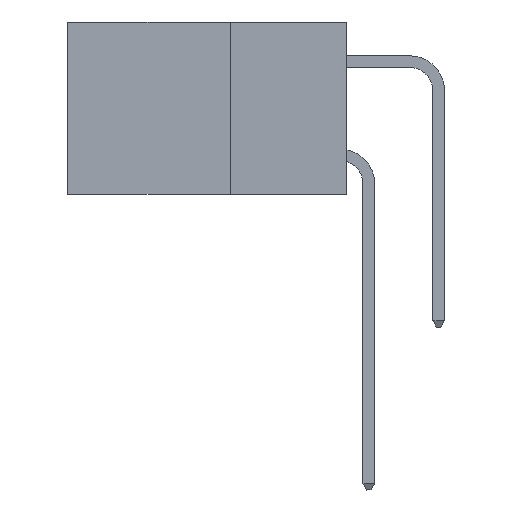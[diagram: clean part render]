
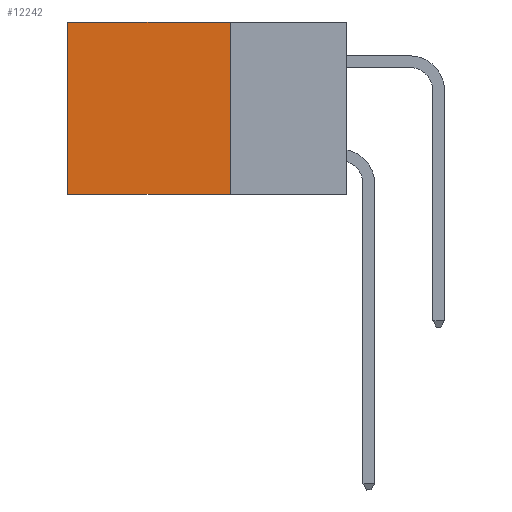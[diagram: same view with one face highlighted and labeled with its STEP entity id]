
A CAD part, left-side view. The second image highlights one B-rep face of the part: STEP entity #12242.
In plain terms, the highlighted planar face has unit normal (-1, 0, 0).
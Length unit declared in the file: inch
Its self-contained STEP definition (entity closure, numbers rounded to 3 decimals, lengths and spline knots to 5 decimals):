
#131 = VERTEX_POINT ( 'NONE', #12599 ) ;
#563 = CARTESIAN_POINT ( 'NONE',  ( 0.2875, 0.25, 0. ) ) ;
#2231 = EDGE_CURVE ( 'NONE', #131, #17688, #21309, .T. ) ;
#2448 = CARTESIAN_POINT ( 'NONE',  ( 0.2875, 0.6, 0. ) ) ;
#2925 = DIRECTION ( 'NONE',  ( 1., 0., 0. ) ) ;
#4211 = CARTESIAN_POINT ( 'NONE',  ( 0.2875, 0.25, -0.37 ) ) ;
#4429 = DIRECTION ( 'NONE',  ( 0., 1., 0. ) ) ;
#4954 = CARTESIAN_POINT ( 'NONE',  ( 0.2875, 0.6, 0. ) ) ;
#5020 = ORIENTED_EDGE ( 'NONE', *, *, #8419, .F. ) ;
#5075 = VECTOR ( 'NONE', #9250, 39.37008 ) ;
#5303 = VERTEX_POINT ( 'NONE', #2448 ) ;
#6988 = AXIS2_PLACEMENT_3D ( 'NONE', #13249, #2925, #16653 ) ;
#8419 = EDGE_CURVE ( 'NONE', #17688, #12035, #9409, .T. ) ;
#9250 = DIRECTION ( 'NONE',  ( 0., 1., 0. ) ) ;
#9409 = LINE ( 'NONE', #4211, #19866 ) ;
#9871 = DIRECTION ( 'NONE',  ( 0., 0., -1. ) ) ;
#10465 = LINE ( 'NONE', #4954, #19599 ) ;
#12035 = VERTEX_POINT ( 'NONE', #17342 ) ;
#12242 = ADVANCED_FACE ( 'NONE', ( #13511 ), #12886, .F. ) ;
#12599 = CARTESIAN_POINT ( 'NONE',  ( 0.2875, 0.25, 0. ) ) ;
#12812 = CARTESIAN_POINT ( 'NONE',  ( 0.2875, 0.25, 0. ) ) ;
#12886 = PLANE ( 'NONE',  #6988 ) ;
#13249 = CARTESIAN_POINT ( 'NONE',  ( 0.2875, 0.25, 0. ) ) ;
#13511 = FACE_OUTER_BOUND ( 'NONE', #13797, .T. ) ;
#13679 = LINE ( 'NONE', #563, #5075 ) ;
#13797 = EDGE_LOOP ( 'NONE', ( #19868, #5020, #19146, #21320 ) ) ;
#14119 = EDGE_CURVE ( 'NONE', #5303, #12035, #10465, .T. ) ;
#16653 = DIRECTION ( 'NONE',  ( 0., 0., -1. ) ) ;
#16944 = EDGE_CURVE ( 'NONE', #131, #5303, #13679, .T. ) ;
#17342 = CARTESIAN_POINT ( 'NONE',  ( 0.2875, 0.6, -0.37 ) ) ;
#17688 = VERTEX_POINT ( 'NONE', #18794 ) ;
#17938 = DIRECTION ( 'NONE',  ( 0., 0., -1. ) ) ;
#18794 = CARTESIAN_POINT ( 'NONE',  ( 0.2875, 0.25, -0.37 ) ) ;
#18859 = VECTOR ( 'NONE', #17938, 39.37008 ) ;
#19146 = ORIENTED_EDGE ( 'NONE', *, *, #2231, .F. ) ;
#19599 = VECTOR ( 'NONE', #9871, 39.37008 ) ;
#19866 = VECTOR ( 'NONE', #4429, 39.37008 ) ;
#19868 = ORIENTED_EDGE ( 'NONE', *, *, #14119, .T. ) ;
#21309 = LINE ( 'NONE', #12812, #18859 ) ;
#21320 = ORIENTED_EDGE ( 'NONE', *, *, #16944, .T. ) ;
